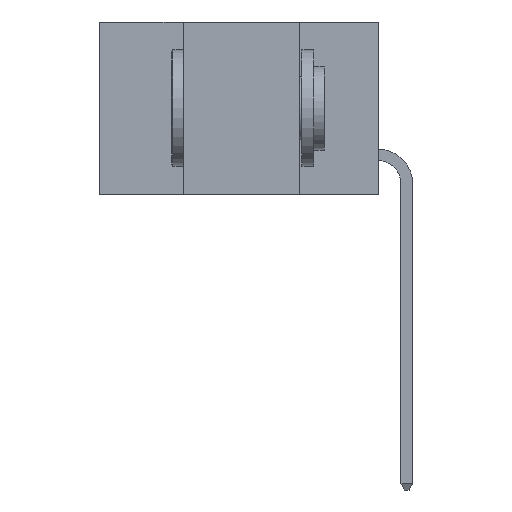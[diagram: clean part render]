
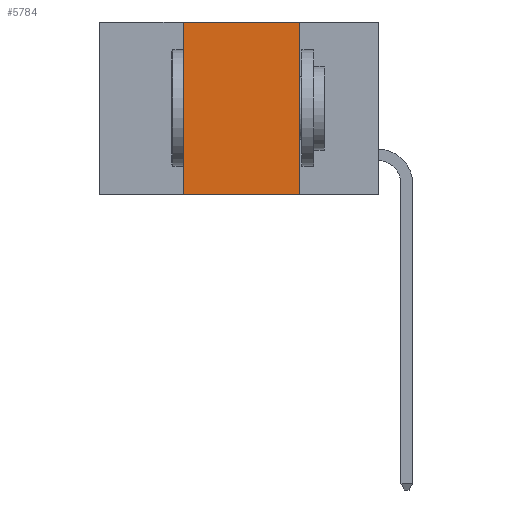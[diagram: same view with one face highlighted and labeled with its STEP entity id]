
A CAD part, left-side view. The second image highlights one B-rep face of the part: STEP entity #5784.
In plain terms, the highlighted planar face has unit normal (-1, 0, 0).
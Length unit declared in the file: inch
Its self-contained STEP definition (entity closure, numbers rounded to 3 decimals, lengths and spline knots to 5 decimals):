
#121 = EDGE_CURVE ( 'NONE', #6279, #418, #8283, .T. ) ;
#323 = EDGE_LOOP ( 'NONE', ( #503, #4067, #1549, #2931 ) ) ;
#365 = VECTOR ( 'NONE', #5703, 39.37008 ) ;
#418 = VERTEX_POINT ( 'NONE', #2980 ) ;
#494 = DIRECTION ( 'NONE',  ( 0., 0., -1. ) ) ;
#503 = ORIENTED_EDGE ( 'NONE', *, *, #4250, .F. ) ;
#623 = LINE ( 'NONE', #6400, #365 ) ;
#1136 = FACE_OUTER_BOUND ( 'NONE', #323, .T. ) ;
#1290 = VERTEX_POINT ( 'NONE', #7285 ) ;
#1549 = ORIENTED_EDGE ( 'NONE', *, *, #6290, .F. ) ;
#2931 = ORIENTED_EDGE ( 'NONE', *, *, #121, .T. ) ;
#2980 = CARTESIAN_POINT ( 'NONE',  ( 0., 0.17, -0.37 ) ) ;
#3292 = LINE ( 'NONE', #6317, #7180 ) ;
#4067 = ORIENTED_EDGE ( 'NONE', *, *, #5365, .F. ) ;
#4250 = EDGE_CURVE ( 'NONE', #1290, #418, #9190, .T. ) ;
#4395 = DIRECTION ( 'NONE',  ( 0., 0., -1. ) ) ;
#4401 = CARTESIAN_POINT ( 'NONE',  ( 0., 0.17, -0.37 ) ) ;
#4437 = PLANE ( 'NONE',  #9465 ) ;
#4541 = CARTESIAN_POINT ( 'NONE',  ( 0., 0.6, -0.37 ) ) ;
#4854 = CARTESIAN_POINT ( 'NONE',  ( 0., 0.42, 0. ) ) ;
#5005 = CARTESIAN_POINT ( 'NONE',  ( 0., 0.42, -0.37 ) ) ;
#5192 = DIRECTION ( 'NONE',  ( 1., 0., 0. ) ) ;
#5365 = EDGE_CURVE ( 'NONE', #7339, #1290, #3292, .T. ) ;
#5703 = DIRECTION ( 'NONE',  ( 0., 0., 1. ) ) ;
#5784 = ADVANCED_FACE ( 'NONE', ( #1136 ), #4437, .F. ) ;
#5802 = DIRECTION ( 'NONE',  ( 0., -1., 0. ) ) ;
#5923 = VECTOR ( 'NONE', #5802, 39.37008 ) ;
#6149 = DIRECTION ( 'NONE',  ( 0., -1., 0. ) ) ;
#6279 = VERTEX_POINT ( 'NONE', #5005 ) ;
#6290 = EDGE_CURVE ( 'NONE', #6279, #7339, #623, .T. ) ;
#6317 = CARTESIAN_POINT ( 'NONE',  ( 0., 0.6, 0. ) ) ;
#6400 = CARTESIAN_POINT ( 'NONE',  ( 0., 0.42, -0.37 ) ) ;
#7180 = VECTOR ( 'NONE', #6149, 39.37008 ) ;
#7285 = CARTESIAN_POINT ( 'NONE',  ( 0., 0.17, 0. ) ) ;
#7316 = VECTOR ( 'NONE', #4395, 39.37008 ) ;
#7339 = VERTEX_POINT ( 'NONE', #4854 ) ;
#8283 = LINE ( 'NONE', #4541, #5923 ) ;
#9190 = LINE ( 'NONE', #4401, #7316 ) ;
#9426 = CARTESIAN_POINT ( 'NONE',  ( 0., 0.6, 0. ) ) ;
#9465 = AXIS2_PLACEMENT_3D ( 'NONE', #9426, #5192, #494 ) ;
